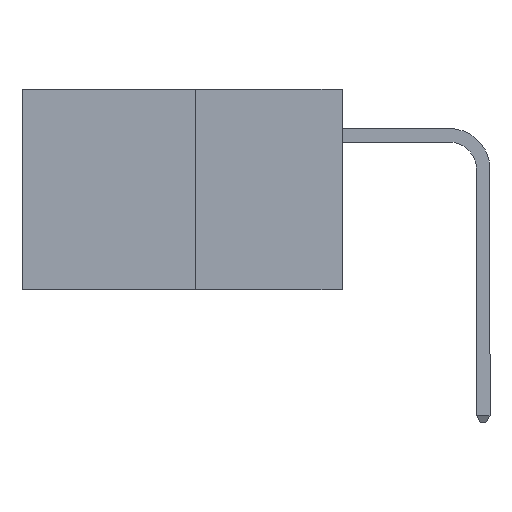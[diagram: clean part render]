
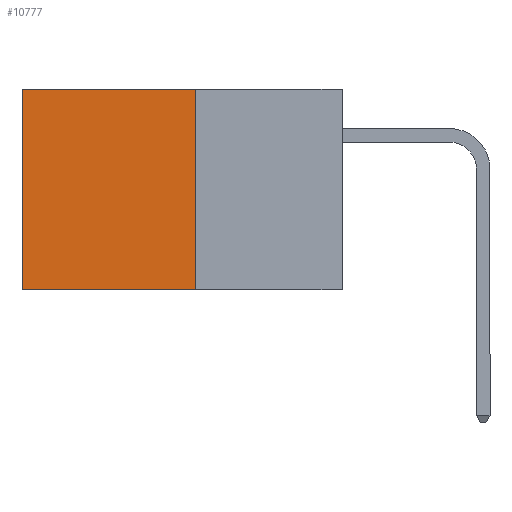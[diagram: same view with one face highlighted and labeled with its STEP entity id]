
A CAD part, left-side view. The second image highlights one B-rep face of the part: STEP entity #10777.
In plain terms, the highlighted planar face has unit normal (-1, 0, 0).
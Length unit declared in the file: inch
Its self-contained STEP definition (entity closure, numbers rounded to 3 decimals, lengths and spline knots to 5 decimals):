
#1039 = VECTOR ( 'NONE', #1534, 39.37008 ) ;
#1254 = VECTOR ( 'NONE', #2184, 39.37008 ) ;
#1534 = DIRECTION ( 'NONE',  ( 0., 0., -1. ) ) ;
#1890 = CARTESIAN_POINT ( 'NONE',  ( 0.277, 0.59, -0.37 ) ) ;
#2184 = DIRECTION ( 'NONE',  ( 0., 0., -1. ) ) ;
#2937 = VERTEX_POINT ( 'NONE', #1890 ) ;
#2963 = LINE ( 'NONE', #9250, #7172 ) ;
#3290 = DIRECTION ( 'NONE',  ( 1., 0., 0. ) ) ;
#3387 = EDGE_CURVE ( 'NONE', #7020, #2937, #2963, .T. ) ;
#3641 = LINE ( 'NONE', #7875, #1039 ) ;
#3714 = EDGE_CURVE ( 'NONE', #6759, #2937, #8494, .T. ) ;
#4152 = VECTOR ( 'NONE', #6520, 39.37008 ) ;
#4288 = CARTESIAN_POINT ( 'NONE',  ( 0.277, 0.27, 0. ) ) ;
#5022 = CARTESIAN_POINT ( 'NONE',  ( 0.277, 0.59, 0. ) ) ;
#5966 = PLANE ( 'NONE',  #9613 ) ;
#6397 = ORIENTED_EDGE ( 'NONE', *, *, #7457, .F. ) ;
#6520 = DIRECTION ( 'NONE',  ( 0., 1., 0. ) ) ;
#6621 = EDGE_LOOP ( 'NONE', ( #7722, #7176, #6397, #6942 ) ) ;
#6759 = VERTEX_POINT ( 'NONE', #5022 ) ;
#6942 = ORIENTED_EDGE ( 'NONE', *, *, #9475, .T. ) ;
#7020 = VERTEX_POINT ( 'NONE', #8153 ) ;
#7172 = VECTOR ( 'NONE', #10235, 39.37008 ) ;
#7176 = ORIENTED_EDGE ( 'NONE', *, *, #3387, .F. ) ;
#7457 = EDGE_CURVE ( 'NONE', #9138, #7020, #3641, .T. ) ;
#7612 = CARTESIAN_POINT ( 'NONE',  ( 0.277, 0.59, -0.37 ) ) ;
#7722 = ORIENTED_EDGE ( 'NONE', *, *, #3714, .T. ) ;
#7875 = CARTESIAN_POINT ( 'NONE',  ( 0.277, 0.27, -0.37 ) ) ;
#8153 = CARTESIAN_POINT ( 'NONE',  ( 0.277, 0.27, -0.37 ) ) ;
#8494 = LINE ( 'NONE', #7612, #1254 ) ;
#8555 = CARTESIAN_POINT ( 'NONE',  ( 0.277, 0.27, -0.37 ) ) ;
#9138 = VERTEX_POINT ( 'NONE', #4288 ) ;
#9250 = CARTESIAN_POINT ( 'NONE',  ( 0.277, 0.27, -0.37 ) ) ;
#9313 = LINE ( 'NONE', #9933, #4152 ) ;
#9407 = DIRECTION ( 'NONE',  ( 0., 0., -1. ) ) ;
#9475 = EDGE_CURVE ( 'NONE', #9138, #6759, #9313, .T. ) ;
#9613 = AXIS2_PLACEMENT_3D ( 'NONE', #8555, #3290, #9407 ) ;
#9933 = CARTESIAN_POINT ( 'NONE',  ( 0.277, 0.27, 0. ) ) ;
#10235 = DIRECTION ( 'NONE',  ( 0., 1., 0. ) ) ;
#10700 = FACE_OUTER_BOUND ( 'NONE', #6621, .T. ) ;
#10777 = ADVANCED_FACE ( 'NONE', ( #10700 ), #5966, .F. ) ;
